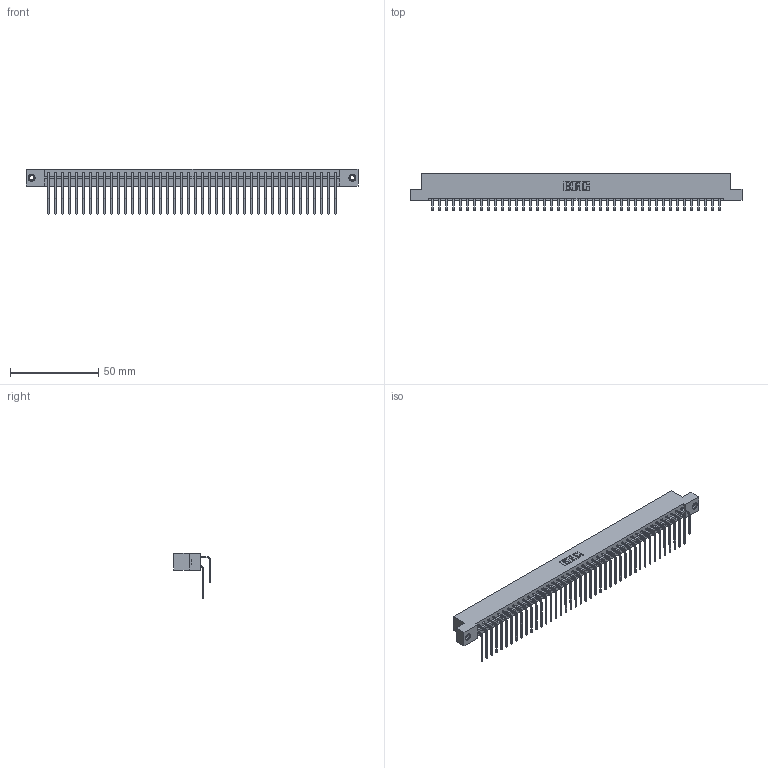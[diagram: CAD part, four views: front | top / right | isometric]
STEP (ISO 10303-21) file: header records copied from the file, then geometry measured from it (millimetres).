
FILE_DESCRIPTION (( 'STEP AP203' ), '1' );
FILE_NAME ('333-084-559-207.STEP', '2018-08-05T05:18:03', ( '' ), ( '' ), 'SwSTEP 2.0', 'SolidWorks 2016', '' );
FILE_SCHEMA (( 'CONFIG_CONTROL_DESIGN' ));
Length unit declared in the file: inch
Products named in the file (5): 345-292-001_558 559 Tail - 1; 345-292-001_559 Tail - 2; 345-250-001_345-250-005-103; 333-084-559-207; 333 Part_Flush - .156 Dia - TI
Assembly tree (87 placements, depth 2):
  333-084-559-207
    333 Part_Flush - .156 Dia - TI
    345-292-001_558 559 Tail - 1  x42
    345-292-001_559 Tail - 2  x42
    345-250-001_345-250-005-103  x2
Bounding box: 187.96 x 20.9 x 25.53 mm (x, y, z)
Volume: 19660.7 mm3; surface area: 25691.6 mm2
Topology: 87 solids, 87 shells, 4710 faces, 13971 edges, 9194 vertices
Faces by surface type: plane 3294, cylinder 1400, cone 12, torus 4
Entity records: 29990 total; most frequent: CARTESIAN_POINT 5004, ORIENTED_EDGE 4882, DIRECTION 4287, EDGE_CURVE 2441, LINE 2253, VECTOR 2253, VERTEX_POINT 1620, AXIS2_PLACEMENT_3D 1017
